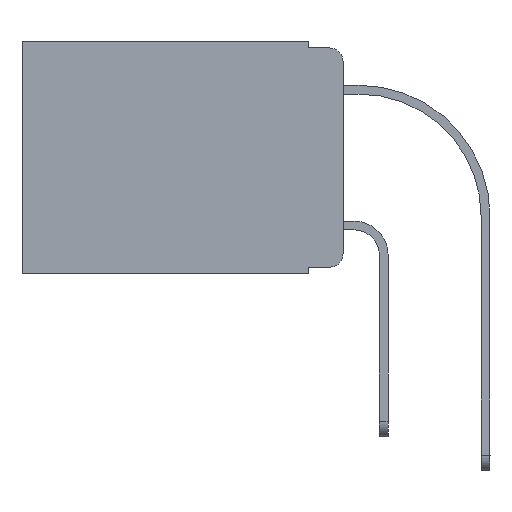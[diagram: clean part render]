
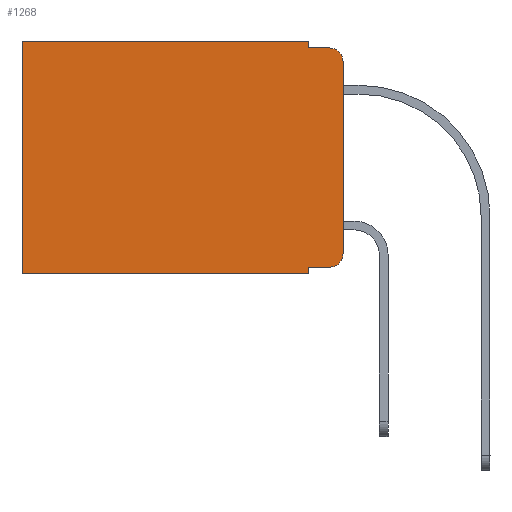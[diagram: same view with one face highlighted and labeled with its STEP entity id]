
A CAD part, left-side view. The second image highlights one B-rep face of the part: STEP entity #1268.
In plain terms, the highlighted planar face has unit normal (-1, 0, 0).
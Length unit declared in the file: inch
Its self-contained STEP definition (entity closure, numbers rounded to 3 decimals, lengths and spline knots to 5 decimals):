
#403 = VERTEX_POINT ( 'NONE', #9943 ) ;
#636 = CARTESIAN_POINT ( 'NONE',  ( 0.298, 0., -0.03 ) ) ;
#686 = VECTOR ( 'NONE', #16183, 39.37008 ) ;
#771 = EDGE_CURVE ( 'NONE', #6573, #1220, #1639, .T. ) ;
#851 = ORIENTED_EDGE ( 'NONE', *, *, #10301, .T. ) ;
#1012 = LINE ( 'NONE', #5237, #13831 ) ;
#1220 = VERTEX_POINT ( 'NONE', #5640 ) ;
#1268 = ADVANCED_FACE ( 'NONE', ( #13519 ), #8309, .F. ) ;
#1403 = ORIENTED_EDGE ( 'NONE', *, *, #15054, .F. ) ;
#1639 = LINE ( 'NONE', #4308, #6910 ) ;
#1884 = VERTEX_POINT ( 'NONE', #14379 ) ;
#2151 = AXIS2_PLACEMENT_3D ( 'NONE', #12300, #16291, #9708 ) ;
#2201 = AXIS2_PLACEMENT_3D ( 'NONE', #16422, #7149, #5693 ) ;
#2499 = VERTEX_POINT ( 'NONE', #12514 ) ;
#3363 = CARTESIAN_POINT ( 'NONE',  ( 0.298, 0., 0. ) ) ;
#3579 = ORIENTED_EDGE ( 'NONE', *, *, #4636, .F. ) ;
#3641 = VECTOR ( 'NONE', #12053, 39.37008 ) ;
#4308 = CARTESIAN_POINT ( 'NONE',  ( 0.298, 0.051, -0.333 ) ) ;
#4339 = LINE ( 'NONE', #16273, #686 ) ;
#4505 = VECTOR ( 'NONE', #5727, 39.37008 ) ;
#4604 = EDGE_LOOP ( 'NONE', ( #1403, #16324, #16010, #10479, #851, #5424, #10519, #3579, #16695, #16440 ) ) ;
#4636 = EDGE_CURVE ( 'NONE', #6573, #13293, #11093, .T. ) ;
#5237 = CARTESIAN_POINT ( 'NONE',  ( 0.298, 0., 0. ) ) ;
#5424 = ORIENTED_EDGE ( 'NONE', *, *, #14511, .T. ) ;
#5640 = CARTESIAN_POINT ( 'NONE',  ( 0.298, 0.02, -0.333 ) ) ;
#5693 = DIRECTION ( 'NONE',  ( 0., 0., -1. ) ) ;
#5727 = DIRECTION ( 'NONE',  ( 0., 0., -1. ) ) ;
#6147 = VERTEX_POINT ( 'NONE', #15607 ) ;
#6573 = VERTEX_POINT ( 'NONE', #13309 ) ;
#6910 = VECTOR ( 'NONE', #9669, 39.37008 ) ;
#7149 = DIRECTION ( 'NONE',  ( -1., 0., 0. ) ) ;
#7172 = VERTEX_POINT ( 'NONE', #16139 ) ;
#7263 = VECTOR ( 'NONE', #10969, 39.37008 ) ;
#7354 = EDGE_CURVE ( 'NONE', #12369, #2499, #13326, .T. ) ;
#7476 = CARTESIAN_POINT ( 'NONE',  ( 0.298, 0., -0.343 ) ) ;
#7571 = EDGE_CURVE ( 'NONE', #7172, #2499, #8399, .T. ) ;
#8299 = LINE ( 'NONE', #10906, #13573 ) ;
#8309 = PLANE ( 'NONE',  #2151 ) ;
#8399 = LINE ( 'NONE', #11012, #3641 ) ;
#8848 = CARTESIAN_POINT ( 'NONE',  ( 0.298, 0.473, -0.343 ) ) ;
#9114 = DIRECTION ( 'NONE',  ( -1., 0., 0. ) ) ;
#9357 = EDGE_CURVE ( 'NONE', #6147, #7172, #8299, .T. ) ;
#9669 = DIRECTION ( 'NONE',  ( 0., -1., 0. ) ) ;
#9708 = DIRECTION ( 'NONE',  ( 0., 0., -1. ) ) ;
#9943 = CARTESIAN_POINT ( 'NONE',  ( 0.298, 0., -0.313 ) ) ;
#10002 = VECTOR ( 'NONE', #12769, 39.37008 ) ;
#10162 = EDGE_CURVE ( 'NONE', #13293, #11948, #16409, .T. ) ;
#10301 = EDGE_CURVE ( 'NONE', #6147, #1884, #1012, .T. ) ;
#10479 = ORIENTED_EDGE ( 'NONE', *, *, #9357, .F. ) ;
#10519 = ORIENTED_EDGE ( 'NONE', *, *, #10162, .F. ) ;
#10710 = CIRCLE ( 'NONE', #2201, 0.02 ) ;
#10906 = CARTESIAN_POINT ( 'NONE',  ( 0.298, 0.051, 0. ) ) ;
#10969 = DIRECTION ( 'NONE',  ( 0., 0., -1. ) ) ;
#11012 = CARTESIAN_POINT ( 'NONE',  ( 0.298, 0.051, -0.01 ) ) ;
#11093 = LINE ( 'NONE', #16374, #4505 ) ;
#11948 = VERTEX_POINT ( 'NONE', #8848 ) ;
#12053 = DIRECTION ( 'NONE',  ( 0., -1., 0. ) ) ;
#12300 = CARTESIAN_POINT ( 'NONE',  ( 0.298, 0., 0. ) ) ;
#12369 = VERTEX_POINT ( 'NONE', #636 ) ;
#12514 = CARTESIAN_POINT ( 'NONE',  ( 0.298, 0.02, -0.01 ) ) ;
#12769 = DIRECTION ( 'NONE',  ( 0., 1., 0. ) ) ;
#13293 = VERTEX_POINT ( 'NONE', #16395 ) ;
#13309 = CARTESIAN_POINT ( 'NONE',  ( 0.298, 0.051, -0.333 ) ) ;
#13326 = CIRCLE ( 'NONE', #15546, 0.02 ) ;
#13519 = FACE_OUTER_BOUND ( 'NONE', #4604, .T. ) ;
#13573 = VECTOR ( 'NONE', #16187, 39.37008 ) ;
#13831 = VECTOR ( 'NONE', #14233, 39.37008 ) ;
#13996 = LINE ( 'NONE', #3363, #7263 ) ;
#14233 = DIRECTION ( 'NONE',  ( 0., 1., 0. ) ) ;
#14379 = CARTESIAN_POINT ( 'NONE',  ( 0.298, 0.473, 0. ) ) ;
#14475 = CARTESIAN_POINT ( 'NONE',  ( 0.298, 0.02, -0.03 ) ) ;
#14511 = EDGE_CURVE ( 'NONE', #1884, #11948, #4339, .T. ) ;
#15054 = EDGE_CURVE ( 'NONE', #12369, #403, #13996, .T. ) ;
#15122 = EDGE_CURVE ( 'NONE', #1220, #403, #10710, .T. ) ;
#15546 = AXIS2_PLACEMENT_3D ( 'NONE', #14475, #9114, #15697 ) ;
#15607 = CARTESIAN_POINT ( 'NONE',  ( 0.298, 0.051, 0. ) ) ;
#15697 = DIRECTION ( 'NONE',  ( 0., 0., -1. ) ) ;
#16010 = ORIENTED_EDGE ( 'NONE', *, *, #7571, .F. ) ;
#16139 = CARTESIAN_POINT ( 'NONE',  ( 0.298, 0.051, -0.01 ) ) ;
#16183 = DIRECTION ( 'NONE',  ( 0., 0., -1. ) ) ;
#16187 = DIRECTION ( 'NONE',  ( 0., 0., -1. ) ) ;
#16273 = CARTESIAN_POINT ( 'NONE',  ( 0.298, 0.473, 0. ) ) ;
#16291 = DIRECTION ( 'NONE',  ( 1., 0., 0. ) ) ;
#16324 = ORIENTED_EDGE ( 'NONE', *, *, #7354, .T. ) ;
#16374 = CARTESIAN_POINT ( 'NONE',  ( 0.298, 0.051, 0. ) ) ;
#16395 = CARTESIAN_POINT ( 'NONE',  ( 0.298, 0.051, -0.343 ) ) ;
#16409 = LINE ( 'NONE', #7476, #10002 ) ;
#16422 = CARTESIAN_POINT ( 'NONE',  ( 0.298, 0.02, -0.313 ) ) ;
#16440 = ORIENTED_EDGE ( 'NONE', *, *, #15122, .T. ) ;
#16695 = ORIENTED_EDGE ( 'NONE', *, *, #771, .T. ) ;
